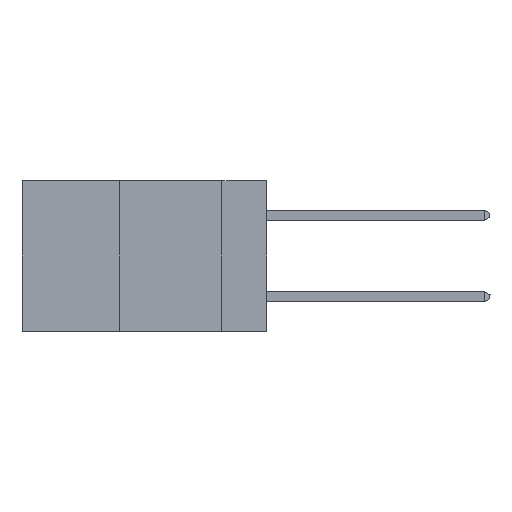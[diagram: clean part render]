
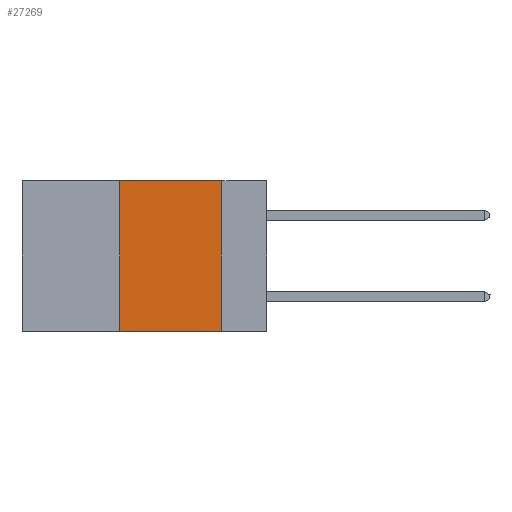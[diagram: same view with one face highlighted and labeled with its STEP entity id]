
A CAD part, left-side view. The second image highlights one B-rep face of the part: STEP entity #27269.
In plain terms, the highlighted planar face has unit normal (-1, 0, 0).
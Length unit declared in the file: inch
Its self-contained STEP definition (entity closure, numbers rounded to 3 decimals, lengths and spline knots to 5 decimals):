
#1234 = EDGE_CURVE ( 'NONE', #14654, #25737, #1749, .T. ) ;
#1749 = LINE ( 'NONE', #6839, #22796 ) ;
#1757 = DIRECTION ( 'NONE',  ( 0., 0., -1. ) ) ;
#2616 = LINE ( 'NONE', #25935, #25648 ) ;
#3907 = VECTOR ( 'NONE', #26074, 39.37008 ) ;
#4872 = AXIS2_PLACEMENT_3D ( 'NONE', #14156, #9821, #22610 ) ;
#5025 = ORIENTED_EDGE ( 'NONE', *, *, #6687, .F. ) ;
#6687 = EDGE_CURVE ( 'NONE', #18460, #13495, #2616, .T. ) ;
#6839 = CARTESIAN_POINT ( 'NONE',  ( 0., 0.6, -0.37 ) ) ;
#7264 = EDGE_CURVE ( 'NONE', #14654, #18460, #12774, .T. ) ;
#8302 = CARTESIAN_POINT ( 'NONE',  ( 0., 0.11, -0.37 ) ) ;
#9821 = DIRECTION ( 'NONE',  ( 1., 0., 0. ) ) ;
#10883 = ORIENTED_EDGE ( 'NONE', *, *, #15675, .F. ) ;
#11586 = CARTESIAN_POINT ( 'NONE',  ( 0., 0.11, 0. ) ) ;
#12017 = PLANE ( 'NONE',  #4872 ) ;
#12170 = DIRECTION ( 'NONE',  ( 0., -1., 0. ) ) ;
#12612 = EDGE_LOOP ( 'NONE', ( #10883, #5025, #19527, #20952 ) ) ;
#12774 = LINE ( 'NONE', #23860, #3907 ) ;
#13495 = VERTEX_POINT ( 'NONE', #11586 ) ;
#13564 = VECTOR ( 'NONE', #1757, 39.37008 ) ;
#14156 = CARTESIAN_POINT ( 'NONE',  ( 0., 0.6, 0. ) ) ;
#14654 = VERTEX_POINT ( 'NONE', #18992 ) ;
#15622 = CARTESIAN_POINT ( 'NONE',  ( 0., 0.36, 0. ) ) ;
#15675 = EDGE_CURVE ( 'NONE', #13495, #25737, #24455, .T. ) ;
#18460 = VERTEX_POINT ( 'NONE', #15622 ) ;
#18779 = CARTESIAN_POINT ( 'NONE',  ( 0., 0.11, 0. ) ) ;
#18992 = CARTESIAN_POINT ( 'NONE',  ( 0., 0.36, -0.37 ) ) ;
#19527 = ORIENTED_EDGE ( 'NONE', *, *, #7264, .F. ) ;
#20952 = ORIENTED_EDGE ( 'NONE', *, *, #1234, .T. ) ;
#21515 = DIRECTION ( 'NONE',  ( 0., -1., 0. ) ) ;
#22610 = DIRECTION ( 'NONE',  ( 0., 0., -1. ) ) ;
#22796 = VECTOR ( 'NONE', #12170, 39.37008 ) ;
#23860 = CARTESIAN_POINT ( 'NONE',  ( 0., 0.36, 0. ) ) ;
#24455 = LINE ( 'NONE', #18779, #13564 ) ;
#25648 = VECTOR ( 'NONE', #21515, 39.37008 ) ;
#25737 = VERTEX_POINT ( 'NONE', #8302 ) ;
#25935 = CARTESIAN_POINT ( 'NONE',  ( 0., 0.6, 0. ) ) ;
#26074 = DIRECTION ( 'NONE',  ( 0., 0., 1. ) ) ;
#26728 = FACE_OUTER_BOUND ( 'NONE', #12612, .T. ) ;
#27269 = ADVANCED_FACE ( 'NONE', ( #26728 ), #12017, .F. ) ;
